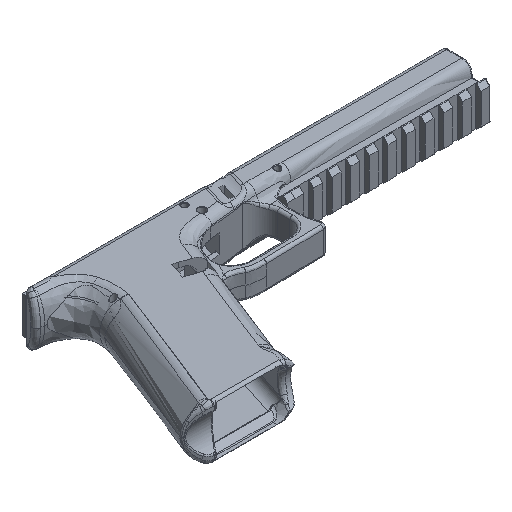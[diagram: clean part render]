
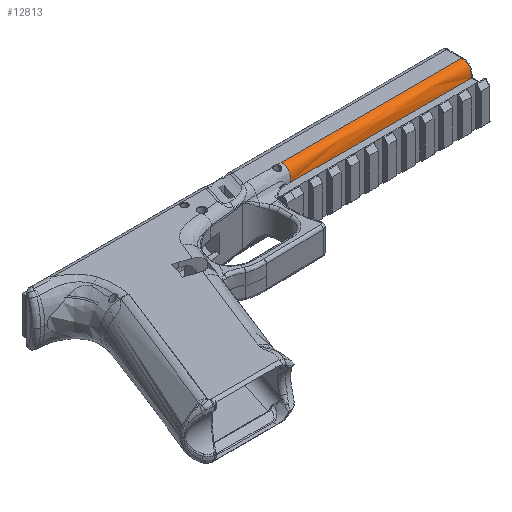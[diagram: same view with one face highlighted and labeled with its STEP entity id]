
A CAD part, isometric view. The second image highlights one B-rep face of the part: STEP entity #12813.
In plain terms, the highlighted free-form (B-spline) face has degree [3, 1] with [12, 2] control points.
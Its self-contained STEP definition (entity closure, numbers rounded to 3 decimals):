
#831=B_SPLINE_SURFACE_WITH_KNOTS('',3,1,((#18063,#18064),(#18065,#18066),
(#18067,#18068),(#18069,#18070),(#18071,#18072),(#18073,#18074),(#18075,
#18076),(#18077,#18078),(#18079,#18080),(#18081,#18082),(#18083,#18084),
(#18085,#18086)),.UNSPECIFIED.,.F.,.F.,.F.,(4,2,2,2,2,4),(2,2),(-0.851,
-0.696,-0.521,-0.371,-0.226,
0.),(0.,9.8),.UNSPECIFIED.);
#985=B_SPLINE_CURVE_WITH_KNOTS('',3,(#17802,#17803,#17804,#17805,#17806,
#17807),.UNSPECIFIED.,.F.,.F.,(4,2,4),(-9.8,-4.9,
-0.1),.UNSPECIFIED.);
#994=B_SPLINE_CURVE_WITH_KNOTS('',3,(#18025,#18026,#18027,#18028,#18029,
#18030,#18031,#18032,#18033,#18034,#18035,#18036,#18037,#18038,#18039,#18040,
#18041,#18042,#18043,#18044,#18045,#18046,#18047,#18048,#18049,#18050,#18051,
#18052),.UNSPECIFIED.,.F.,.F.,(4,2,2,2,2,2,2,2,2,2,2,2,2,4),(0.,
0.071,0.137,0.194,0.246,
0.303,0.367,0.435,0.505,
0.576,0.647,0.718,0.791,
0.811),.UNSPECIFIED.);
#995=B_SPLINE_CURVE_WITH_KNOTS('',3,(#18091,#18092,#18093,#18094,#18095,
#18096,#18097,#18098,#18099,#18100,#18101,#18102,#18103,#18104,#18105,#18106),
 .UNSPECIFIED.,.F.,.F.,(4,3,3,3,3,4),(-0.816,-0.696,
-0.521,-0.371,-0.226,0.),
 .UNSPECIFIED.);
#1526=FACE_OUTER_BOUND('',#2265,.T.);
#2265=EDGE_LOOP('',(#8532,#8533,#8534,#8535,#8536));
#3048=LINE('',#18088,#4065);
#3049=LINE('',#18090,#4066);
#4065=VECTOR('',#14673,10.);
#4066=VECTOR('',#14674,10.);
#5080=VERTEX_POINT('',#17784);
#5081=VERTEX_POINT('',#17801);
#5092=VERTEX_POINT('',#17872);
#5093=VERTEX_POINT('',#18087);
#5094=VERTEX_POINT('',#18089);
#6404=EDGE_CURVE('',#5081,#5080,#985,.T.);
#6420=EDGE_CURVE('',#5092,#5080,#994,.T.);
#6422=EDGE_CURVE('',#5093,#5092,#3048,.T.);
#6423=EDGE_CURVE('',#5094,#5093,#3049,.T.);
#6424=EDGE_CURVE('',#5081,#5094,#995,.T.);
#8532=ORIENTED_EDGE('',*,*,#6420,.F.);
#8533=ORIENTED_EDGE('',*,*,#6422,.F.);
#8534=ORIENTED_EDGE('',*,*,#6423,.F.);
#8535=ORIENTED_EDGE('',*,*,#6424,.F.);
#8536=ORIENTED_EDGE('',*,*,#6404,.T.);
#12813=ADVANCED_FACE('',(#1526),#831,.F.);
#14673=DIRECTION('',(1.,0.,0.));
#14674=DIRECTION('',(1.,0.,0.));
#17784=CARTESIAN_POINT('',(223.,-16.992,7.818));
#17801=CARTESIAN_POINT('',(126.,-16.992,7.818));
#17802=CARTESIAN_POINT('Ctrl Pts',(126.,-16.992,7.818));
#17803=CARTESIAN_POINT('Ctrl Pts',(142.333,-16.992,7.818));
#17804=CARTESIAN_POINT('Ctrl Pts',(158.667,-16.992,7.818));
#17805=CARTESIAN_POINT('Ctrl Pts',(191.,-16.992,7.818));
#17806=CARTESIAN_POINT('Ctrl Pts',(207.,-16.992,7.818));
#17807=CARTESIAN_POINT('Ctrl Pts',(223.,-16.992,7.818));
#17872=CARTESIAN_POINT('',(223.,-11.664,14.4));
#18025=CARTESIAN_POINT('Ctrl Pts',(223.,-11.664,14.4));
#18026=CARTESIAN_POINT('Ctrl Pts',(223.,-11.92,14.397));
#18027=CARTESIAN_POINT('Ctrl Pts',(223.,-12.182,14.386));
#18028=CARTESIAN_POINT('Ctrl Pts',(223.,-12.695,14.34));
#18029=CARTESIAN_POINT('Ctrl Pts',(223.,-12.948,14.308));
#18030=CARTESIAN_POINT('Ctrl Pts',(223.,-13.431,14.212));
#18031=CARTESIAN_POINT('Ctrl Pts',(223.,-13.671,14.152));
#18032=CARTESIAN_POINT('Ctrl Pts',(223.,-14.149,13.969));
#18033=CARTESIAN_POINT('Ctrl Pts',(223.,-14.374,13.855));
#18034=CARTESIAN_POINT('Ctrl Pts',(223.,-14.813,13.557));
#18035=CARTESIAN_POINT('Ctrl Pts',(223.,-15.004,13.387));
#18036=CARTESIAN_POINT('Ctrl Pts',(223.,-15.367,13.01));
#18037=CARTESIAN_POINT('Ctrl Pts',(223.,-15.533,12.8));
#18038=CARTESIAN_POINT('Ctrl Pts',(223.,-15.839,12.354));
#18039=CARTESIAN_POINT('Ctrl Pts',(223.,-15.975,12.118));
#18040=CARTESIAN_POINT('Ctrl Pts',(223.,-16.219,11.632));
#18041=CARTESIAN_POINT('Ctrl Pts',(223.,-16.326,11.382));
#18042=CARTESIAN_POINT('Ctrl Pts',(223.,-16.511,10.875));
#18043=CARTESIAN_POINT('Ctrl Pts',(223.,-16.589,10.619));
#18044=CARTESIAN_POINT('Ctrl Pts',(223.,-16.721,10.107));
#18045=CARTESIAN_POINT('Ctrl Pts',(223.,-16.776,9.848));
#18046=CARTESIAN_POINT('Ctrl Pts',(223.,-16.866,9.331));
#18047=CARTESIAN_POINT('Ctrl Pts',(223.,-16.901,9.072));
#18048=CARTESIAN_POINT('Ctrl Pts',(223.,-16.954,8.551));
#18049=CARTESIAN_POINT('Ctrl Pts',(223.,-16.972,8.29));
#18050=CARTESIAN_POINT('Ctrl Pts',(223.,-16.987,7.96));
#18051=CARTESIAN_POINT('Ctrl Pts',(223.,-16.989,7.889));
#18052=CARTESIAN_POINT('Ctrl Pts',(223.,-16.992,7.818));
#18063=CARTESIAN_POINT('Ctrl Pts',(126.,-17.,7.246));
#18064=CARTESIAN_POINT('Ctrl Pts',(224.002,-17.,7.246));
#18065=CARTESIAN_POINT('Ctrl Pts',(126.,-17.,8.088));
#18066=CARTESIAN_POINT('Ctrl Pts',(224.002,-17.,8.088));
#18067=CARTESIAN_POINT('Ctrl Pts',(126.,-16.951,8.905));
#18068=CARTESIAN_POINT('Ctrl Pts',(224.002,-16.951,8.905));
#18069=CARTESIAN_POINT('Ctrl Pts',(126.,-16.623,10.652));
#18070=CARTESIAN_POINT('Ctrl Pts',(224.002,-16.623,10.652));
#18071=CARTESIAN_POINT('Ctrl Pts',(126.,-16.353,11.404));
#18072=CARTESIAN_POINT('Ctrl Pts',(224.002,-16.353,11.404));
#18073=CARTESIAN_POINT('Ctrl Pts',(126.,-15.728,12.569));
#18074=CARTESIAN_POINT('Ctrl Pts',(224.002,-15.728,12.569));
#18075=CARTESIAN_POINT('Ctrl Pts',(126.,-15.397,13.002));
#18076=CARTESIAN_POINT('Ctrl Pts',(224.002,-15.397,13.002));
#18077=CARTESIAN_POINT('Ctrl Pts',(126.,-14.717,13.652));
#18078=CARTESIAN_POINT('Ctrl Pts',(224.002,-14.717,13.652));
#18079=CARTESIAN_POINT('Ctrl Pts',(126.,-14.354,13.89));
#18080=CARTESIAN_POINT('Ctrl Pts',(224.002,-14.354,13.89));
#18081=CARTESIAN_POINT('Ctrl Pts',(126.,-13.246,14.315));
#18082=CARTESIAN_POINT('Ctrl Pts',(224.002,-13.246,14.315));
#18083=CARTESIAN_POINT('Ctrl Pts',(126.,-12.418,14.39));
#18084=CARTESIAN_POINT('Ctrl Pts',(224.002,-12.418,14.39));
#18085=CARTESIAN_POINT('Ctrl Pts',(126.,-11.664,14.4));
#18086=CARTESIAN_POINT('Ctrl Pts',(224.002,-11.664,14.4));
#18087=CARTESIAN_POINT('',(183.,-11.664,14.4));
#18088=CARTESIAN_POINT('',(183.,-11.664,14.4));
#18089=CARTESIAN_POINT('',(126.,-11.664,14.4));
#18090=CARTESIAN_POINT('',(126.,-11.664,14.4));
#18091=CARTESIAN_POINT('Ctrl Pts',(126.,-16.992,7.818));
#18092=CARTESIAN_POINT('Ctrl Pts',(126.,-16.972,8.461));
#18093=CARTESIAN_POINT('Ctrl Pts',(126.,-16.915,9.092));
#18094=CARTESIAN_POINT('Ctrl Pts',(126.,-16.796,9.728));
#18095=CARTESIAN_POINT('Ctrl Pts',(126.,-16.623,10.652));
#18096=CARTESIAN_POINT('Ctrl Pts',(126.,-16.353,11.404));
#18097=CARTESIAN_POINT('Ctrl Pts',(126.,-16.017,12.031));
#18098=CARTESIAN_POINT('Ctrl Pts',(126.,-15.728,12.569));
#18099=CARTESIAN_POINT('Ctrl Pts',(126.,-15.397,13.002));
#18100=CARTESIAN_POINT('Ctrl Pts',(126.,-15.051,13.333));
#18101=CARTESIAN_POINT('Ctrl Pts',(126.,-14.717,13.652));
#18102=CARTESIAN_POINT('Ctrl Pts',(126.,-14.354,13.89));
#18103=CARTESIAN_POINT('Ctrl Pts',(126.,-13.922,14.056));
#18104=CARTESIAN_POINT('Ctrl Pts',(126.,-13.246,14.315));
#18105=CARTESIAN_POINT('Ctrl Pts',(126.,-12.418,14.39));
#18106=CARTESIAN_POINT('Ctrl Pts',(126.,-11.664,14.4));
